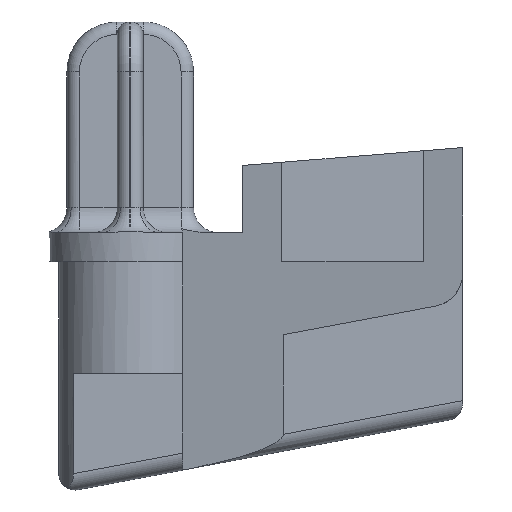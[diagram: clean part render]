
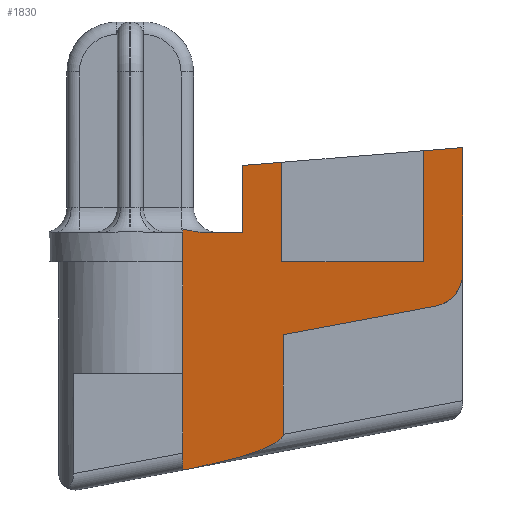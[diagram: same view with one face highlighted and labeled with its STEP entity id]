
A CAD part, left-side view. The second image highlights one B-rep face of the part: STEP entity #1830.
In plain terms, the highlighted planar face has unit normal (-0.982, 0.187, 0).
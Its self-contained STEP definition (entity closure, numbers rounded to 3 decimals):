
#34=PLANE('',#2030);
#63=B_SPLINE_CURVE_WITH_KNOTS('',3,(#2805,#2806,#2807,#2808,#2809,#2810),
 .UNSPECIFIED.,.F.,.F.,(4,2,4),(0.036,0.109,0.167),
 .UNSPECIFIED.);
#92=ELLIPSE('',#2028,5.439,1.);
#94=ELLIPSE('',#2031,2.036,2.);
#121=LINE('',#2967,#270);
#160=LINE('',#3141,#309);
#170=LINE('',#3160,#319);
#176=LINE('',#3179,#325);
#190=LINE('',#3215,#339);
#191=LINE('',#3217,#340);
#192=LINE('',#3220,#341);
#193=LINE('',#3222,#342);
#194=LINE('',#3224,#343);
#195=LINE('',#3226,#344);
#196=LINE('',#3228,#345);
#197=LINE('',#3229,#346);
#270=VECTOR('',#2303,10.);
#309=VECTOR('',#2416,10.);
#319=VECTOR('',#2428,10.);
#325=VECTOR('',#2444,10.);
#339=VECTOR('',#2476,10.);
#340=VECTOR('',#2477,10.);
#341=VECTOR('',#2480,10.);
#342=VECTOR('',#2481,10.);
#343=VECTOR('',#2482,10.);
#344=VECTOR('',#2483,10.);
#345=VECTOR('',#2484,10.);
#346=VECTOR('',#2485,10.);
#494=FACE_OUTER_BOUND('',#604,.T.);
#604=EDGE_LOOP('',(#1480,#1481,#1482,#1483,#1484,#1485,#1486,#1487,#1488,
#1489,#1490,#1491,#1492,#1493,#1494));
#777=VERTEX_POINT('',#2803);
#778=VERTEX_POINT('',#2804);
#809=VERTEX_POINT('',#2966);
#848=VERTEX_POINT('',#3139);
#856=VERTEX_POINT('',#3158);
#863=VERTEX_POINT('',#3176);
#864=VERTEX_POINT('',#3178);
#876=VERTEX_POINT('',#3209);
#877=VERTEX_POINT('',#3214);
#878=VERTEX_POINT('',#3216);
#879=VERTEX_POINT('',#3219);
#880=VERTEX_POINT('',#3221);
#881=VERTEX_POINT('',#3223);
#882=VERTEX_POINT('',#3225);
#883=VERTEX_POINT('',#3227);
#955=EDGE_CURVE('',#777,#778,#63,.F.);
#1006=EDGE_CURVE('',#777,#809,#121,.T.);
#1067=EDGE_CURVE('',#778,#848,#160,.T.);
#1077=EDGE_CURVE('',#848,#856,#170,.T.);
#1086=EDGE_CURVE('',#864,#863,#176,.T.);
#1103=EDGE_CURVE('',#876,#856,#92,.T.);
#1105=EDGE_CURVE('',#876,#877,#190,.T.);
#1106=EDGE_CURVE('',#877,#878,#191,.T.);
#1107=EDGE_CURVE('',#864,#878,#94,.T.);
#1108=EDGE_CURVE('',#879,#863,#192,.T.);
#1109=EDGE_CURVE('',#880,#879,#193,.T.);
#1110=EDGE_CURVE('',#881,#880,#194,.T.);
#1111=EDGE_CURVE('',#881,#882,#195,.T.);
#1112=EDGE_CURVE('',#883,#882,#196,.T.);
#1113=EDGE_CURVE('',#809,#883,#197,.T.);
#1480=ORIENTED_EDGE('',*,*,#1103,.F.);
#1481=ORIENTED_EDGE('',*,*,#1105,.T.);
#1482=ORIENTED_EDGE('',*,*,#1106,.T.);
#1483=ORIENTED_EDGE('',*,*,#1107,.F.);
#1484=ORIENTED_EDGE('',*,*,#1086,.T.);
#1485=ORIENTED_EDGE('',*,*,#1108,.F.);
#1486=ORIENTED_EDGE('',*,*,#1109,.F.);
#1487=ORIENTED_EDGE('',*,*,#1110,.F.);
#1488=ORIENTED_EDGE('',*,*,#1111,.T.);
#1489=ORIENTED_EDGE('',*,*,#1112,.F.);
#1490=ORIENTED_EDGE('',*,*,#1113,.F.);
#1491=ORIENTED_EDGE('',*,*,#1006,.F.);
#1492=ORIENTED_EDGE('',*,*,#955,.T.);
#1493=ORIENTED_EDGE('',*,*,#1067,.T.);
#1494=ORIENTED_EDGE('',*,*,#1077,.T.);
#1830=ADVANCED_FACE('',(#494),#34,.T.);
#2028=AXIS2_PLACEMENT_3D('',#3211,#2470,#2471);
#2030=AXIS2_PLACEMENT_3D('',#3213,#2474,#2475);
#2031=AXIS2_PLACEMENT_3D('',#3218,#2478,#2479);
#2303=DIRECTION('',(-0.187,-0.982,0.));
#2416=DIRECTION('',(0.,0.,-1.));
#2428=DIRECTION('',(-0.184,-0.966,0.181));
#2444=DIRECTION('',(0.,0.,1.));
#2470=DIRECTION('center_axis',(0.982,-0.187,0.));
#2471=DIRECTION('ref_axis',(-0.184,-0.965,0.188));
#2474=DIRECTION('center_axis',(-0.982,0.187,0.));
#2475=DIRECTION('ref_axis',(-0.187,-0.982,0.));
#2476=DIRECTION('',(0.,0.,1.));
#2477=DIRECTION('',(-0.184,-0.966,0.181));
#2478=DIRECTION('center_axis',(0.982,-0.187,0.));
#2479=DIRECTION('ref_axis',(-0.187,-0.982,0.));
#2480=DIRECTION('',(-0.186,-0.979,0.08));
#2481=DIRECTION('',(0.,0.,1.));
#2482=DIRECTION('',(-0.187,-0.982,0.));
#2483=DIRECTION('',(0.,0.,1.));
#2484=DIRECTION('',(-0.186,-0.979,0.08));
#2485=DIRECTION('',(0.,0.,1.));
#2803=CARTESIAN_POINT('',(-7.86,25.238,1.75));
#2804=CARTESIAN_POINT('',(-7.601,26.6,1.978));
#2805=CARTESIAN_POINT('Ctrl Pts',(-7.601,26.6,1.978));
#2806=CARTESIAN_POINT('Ctrl Pts',(-7.649,26.344,1.937));
#2807=CARTESIAN_POINT('Ctrl Pts',(-7.699,26.082,1.863));
#2808=CARTESIAN_POINT('Ctrl Pts',(-7.78,25.658,1.779));
#2809=CARTESIAN_POINT('Ctrl Pts',(-7.824,25.43,1.75));
#2810=CARTESIAN_POINT('Ctrl Pts',(-7.86,25.238,1.75));
#2966=CARTESIAN_POINT('',(-8.286,23.,1.75));
#2967=CARTESIAN_POINT('',(-6.125,34.35,1.75));
#3139=CARTESIAN_POINT('',(-7.601,26.6,-12.502));
#3141=CARTESIAN_POINT('',(-7.601,26.6,0.875));
#3158=CARTESIAN_POINT('',(-7.75,25.817,-12.355));
#3160=CARTESIAN_POINT('',(-8.411,22.346,-11.704));
#3176=CARTESIAN_POINT('',(-10.8,9.8,6.862));
#3178=CARTESIAN_POINT('',(-10.8,9.8,-0.69));
#3179=CARTESIAN_POINT('',(-10.8,9.8,0.));
#3209=CARTESIAN_POINT('',(-8.75,20.565,-10.352));
#3211=CARTESIAN_POINT('Origin',(-7.75,25.817,-11.338));
#3213=CARTESIAN_POINT('Origin',(-10.352,12.15,0.));
#3214=CARTESIAN_POINT('',(-8.75,20.565,-4.37));
#3215=CARTESIAN_POINT('',(-8.75,20.565,-3.615));
#3216=CARTESIAN_POINT('',(-10.489,11.431,-2.656));
#3217=CARTESIAN_POINT('',(-10.575,10.979,-2.571));
#3218=CARTESIAN_POINT('Origin',(-10.419,11.8,-0.69));
#3219=CARTESIAN_POINT('',(-10.352,12.15,6.671));
#3220=CARTESIAN_POINT('',(-8.193,23.489,5.747));
#3221=CARTESIAN_POINT('',(-10.352,12.15,0.));
#3222=CARTESIAN_POINT('',(-10.352,12.15,3.559));
#3223=CARTESIAN_POINT('',(-8.734,20.65,0.));
#3224=CARTESIAN_POINT('',(-8.661,21.03,0.));
#3225=CARTESIAN_POINT('',(-8.734,20.65,5.978));
#3226=CARTESIAN_POINT('',(-8.734,20.65,0.));
#3227=CARTESIAN_POINT('',(-8.286,23.,5.787));
#3228=CARTESIAN_POINT('',(-7.167,28.88,5.308));
#3229=CARTESIAN_POINT('',(-8.286,23.,0.));
